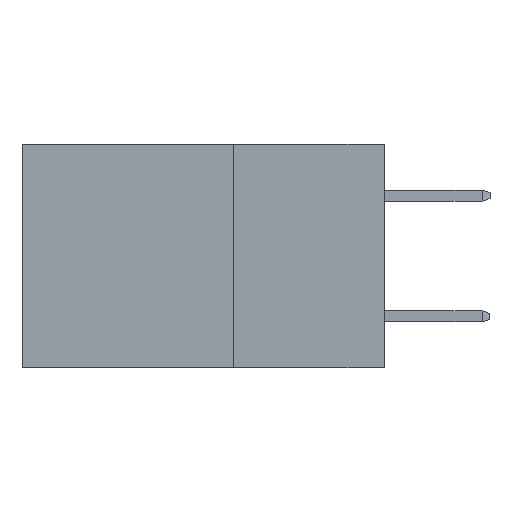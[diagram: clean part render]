
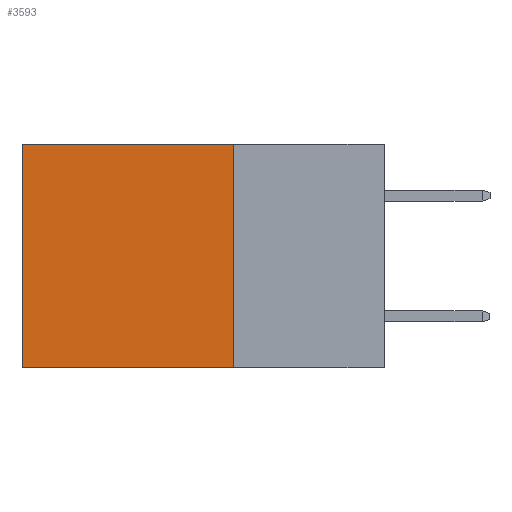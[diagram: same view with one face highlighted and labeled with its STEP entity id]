
A CAD part, left-side view. The second image highlights one B-rep face of the part: STEP entity #3593.
In plain terms, the highlighted planar face has unit normal (-1, 0, 0).
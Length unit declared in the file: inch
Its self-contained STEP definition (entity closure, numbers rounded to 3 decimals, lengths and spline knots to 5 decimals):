
#535 = LINE ( 'NONE', #2226, #10655 ) ;
#550 = DIRECTION ( 'NONE',  ( 0., 1., 0. ) ) ;
#855 = CARTESIAN_POINT ( 'NONE',  ( 0.298, 0.25, -0.37 ) ) ;
#1056 = ORIENTED_EDGE ( 'NONE', *, *, #11251, .T. ) ;
#1068 = AXIS2_PLACEMENT_3D ( 'NONE', #6503, #2583, #9453 ) ;
#1503 = EDGE_CURVE ( 'NONE', #5097, #6848, #10144, .T. ) ;
#1568 = ORIENTED_EDGE ( 'NONE', *, *, #1503, .F. ) ;
#1842 = CARTESIAN_POINT ( 'NONE',  ( 0.298, 0.6, -0.37 ) ) ;
#1960 = ORIENTED_EDGE ( 'NONE', *, *, #3564, .F. ) ;
#2092 = DIRECTION ( 'NONE',  ( 0., 0., -1. ) ) ;
#2226 = CARTESIAN_POINT ( 'NONE',  ( 0.298, 0.6, 0. ) ) ;
#2322 = VECTOR ( 'NONE', #12479, 39.37008 ) ;
#2583 = DIRECTION ( 'NONE',  ( 1., 0., 0. ) ) ;
#2830 = ORIENTED_EDGE ( 'NONE', *, *, #9898, .T. ) ;
#3564 = EDGE_CURVE ( 'NONE', #6848, #4827, #9975, .T. ) ;
#3593 = ADVANCED_FACE ( 'NONE', ( #5786 ), #8446, .F. ) ;
#4402 = CARTESIAN_POINT ( 'NONE',  ( 0.298, 0.25, 0. ) ) ;
#4748 = VECTOR ( 'NONE', #550, 39.37008 ) ;
#4827 = VERTEX_POINT ( 'NONE', #1842 ) ;
#5097 = VERTEX_POINT ( 'NONE', #6287 ) ;
#5770 = VERTEX_POINT ( 'NONE', #11808 ) ;
#5786 = FACE_OUTER_BOUND ( 'NONE', #11442, .T. ) ;
#6254 = CARTESIAN_POINT ( 'NONE',  ( 0.298, 0.25, -0.37 ) ) ;
#6287 = CARTESIAN_POINT ( 'NONE',  ( 0.298, 0.25, 0. ) ) ;
#6503 = CARTESIAN_POINT ( 'NONE',  ( 0.298, 0.25, 0. ) ) ;
#6848 = VERTEX_POINT ( 'NONE', #6254 ) ;
#7362 = VECTOR ( 'NONE', #7725, 39.37008 ) ;
#7363 = LINE ( 'NONE', #4402, #4748 ) ;
#7725 = DIRECTION ( 'NONE',  ( 0., 1., 0. ) ) ;
#8446 = PLANE ( 'NONE',  #1068 ) ;
#9453 = DIRECTION ( 'NONE',  ( 0., 0., -1. ) ) ;
#9898 = EDGE_CURVE ( 'NONE', #5770, #4827, #535, .T. ) ;
#9975 = LINE ( 'NONE', #855, #7362 ) ;
#10144 = LINE ( 'NONE', #11673, #2322 ) ;
#10655 = VECTOR ( 'NONE', #2092, 39.37008 ) ;
#11251 = EDGE_CURVE ( 'NONE', #5097, #5770, #7363, .T. ) ;
#11442 = EDGE_LOOP ( 'NONE', ( #2830, #1960, #1568, #1056 ) ) ;
#11673 = CARTESIAN_POINT ( 'NONE',  ( 0.298, 0.25, 0. ) ) ;
#11808 = CARTESIAN_POINT ( 'NONE',  ( 0.298, 0.6, 0. ) ) ;
#12479 = DIRECTION ( 'NONE',  ( 0., 0., -1. ) ) ;
